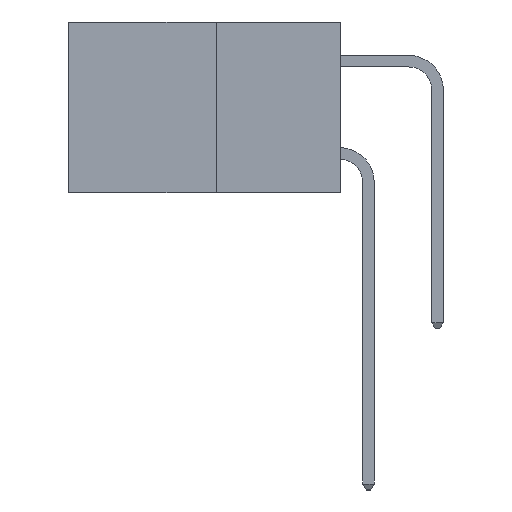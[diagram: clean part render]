
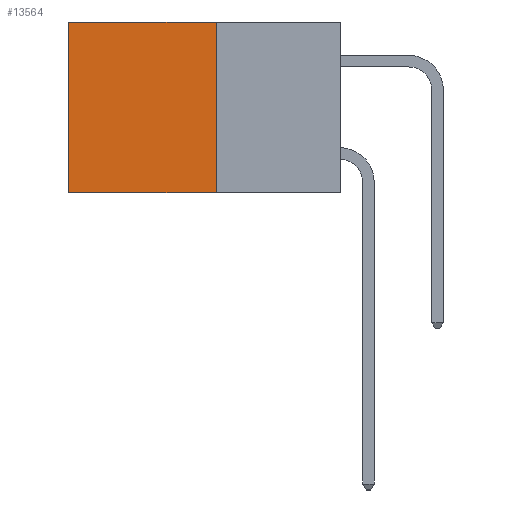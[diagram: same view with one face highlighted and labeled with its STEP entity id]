
A CAD part, left-side view. The second image highlights one B-rep face of the part: STEP entity #13564.
In plain terms, the highlighted planar face has unit normal (-1, 0, 0).
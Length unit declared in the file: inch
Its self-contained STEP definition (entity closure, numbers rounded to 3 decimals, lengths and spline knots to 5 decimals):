
#587 = VECTOR ( 'NONE', #4350, 39.37008 ) ;
#637 = VECTOR ( 'NONE', #1698, 39.37008 ) ;
#917 = DIRECTION ( 'NONE',  ( 0., 1., 0. ) ) ;
#962 = FACE_OUTER_BOUND ( 'NONE', #9065, .T. ) ;
#1558 = EDGE_CURVE ( 'NONE', #12801, #9752, #6343, .T. ) ;
#1698 = DIRECTION ( 'NONE',  ( 0., 0., -1. ) ) ;
#2007 = CARTESIAN_POINT ( 'NONE',  ( 0.277, 0.27, -0.37 ) ) ;
#2058 = DIRECTION ( 'NONE',  ( 0., 0., -1. ) ) ;
#2093 = ORIENTED_EDGE ( 'NONE', *, *, #7637, .T. ) ;
#3663 = ORIENTED_EDGE ( 'NONE', *, *, #7913, .F. ) ;
#3880 = ORIENTED_EDGE ( 'NONE', *, *, #10763, .T. ) ;
#4168 = PLANE ( 'NONE',  #9201 ) ;
#4350 = DIRECTION ( 'NONE',  ( 0., 0., -1. ) ) ;
#5308 = CARTESIAN_POINT ( 'NONE',  ( 0.277, 0.27, -0.37 ) ) ;
#5880 = CARTESIAN_POINT ( 'NONE',  ( 0.277, 0.59, -0.37 ) ) ;
#6343 = LINE ( 'NONE', #2007, #587 ) ;
#6815 = VERTEX_POINT ( 'NONE', #5880 ) ;
#7422 = VECTOR ( 'NONE', #917, 39.37008 ) ;
#7476 = CARTESIAN_POINT ( 'NONE',  ( 0.277, 0.27, 0. ) ) ;
#7637 = EDGE_CURVE ( 'NONE', #9730, #6815, #12200, .T. ) ;
#7913 = EDGE_CURVE ( 'NONE', #9752, #6815, #8541, .T. ) ;
#8541 = LINE ( 'NONE', #12944, #11711 ) ;
#8650 = DIRECTION ( 'NONE',  ( 1., 0., 0. ) ) ;
#9065 = EDGE_LOOP ( 'NONE', ( #2093, #3663, #10996, #3880 ) ) ;
#9201 = AXIS2_PLACEMENT_3D ( 'NONE', #5308, #8650, #2058 ) ;
#9645 = LINE ( 'NONE', #7476, #7422 ) ;
#9730 = VERTEX_POINT ( 'NONE', #10091 ) ;
#9752 = VERTEX_POINT ( 'NONE', #13211 ) ;
#10091 = CARTESIAN_POINT ( 'NONE',  ( 0.277, 0.59, 0. ) ) ;
#10763 = EDGE_CURVE ( 'NONE', #12801, #9730, #9645, .T. ) ;
#10996 = ORIENTED_EDGE ( 'NONE', *, *, #1558, .F. ) ;
#11711 = VECTOR ( 'NONE', #13934, 39.37008 ) ;
#11755 = CARTESIAN_POINT ( 'NONE',  ( 0.277, 0.27, 0. ) ) ;
#12200 = LINE ( 'NONE', #12505, #637 ) ;
#12505 = CARTESIAN_POINT ( 'NONE',  ( 0.277, 0.59, -0.37 ) ) ;
#12801 = VERTEX_POINT ( 'NONE', #11755 ) ;
#12944 = CARTESIAN_POINT ( 'NONE',  ( 0.277, 0.27, -0.37 ) ) ;
#13211 = CARTESIAN_POINT ( 'NONE',  ( 0.277, 0.27, -0.37 ) ) ;
#13564 = ADVANCED_FACE ( 'NONE', ( #962 ), #4168, .F. ) ;
#13934 = DIRECTION ( 'NONE',  ( 0., 1., 0. ) ) ;
